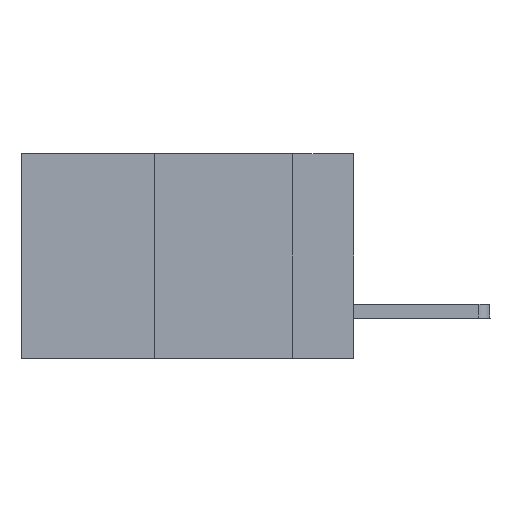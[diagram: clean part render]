
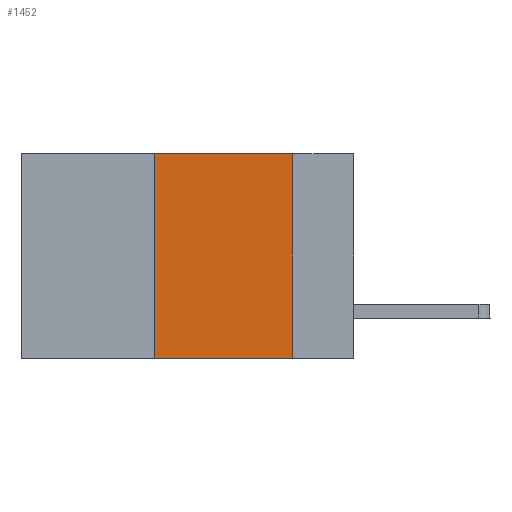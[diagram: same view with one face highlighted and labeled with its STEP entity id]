
A CAD part, left-side view. The second image highlights one B-rep face of the part: STEP entity #1452.
In plain terms, the highlighted planar face has unit normal (-1, 0, 0).
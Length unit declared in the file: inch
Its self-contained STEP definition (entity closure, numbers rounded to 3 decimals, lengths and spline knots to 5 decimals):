
#301 = DIRECTION ( 'NONE',  ( 1., 0., 0. ) ) ;
#927 = VERTEX_POINT ( 'NONE', #1703 ) ;
#1042 = EDGE_CURVE ( 'NONE', #5580, #927, #5784, .T. ) ;
#1264 = LINE ( 'NONE', #8928, #13347 ) ;
#1402 = VERTEX_POINT ( 'NONE', #9039 ) ;
#1452 = ADVANCED_FACE ( 'NONE', ( #6966 ), #12421, .F. ) ;
#1644 = VECTOR ( 'NONE', #13231, 39.37008 ) ;
#1703 = CARTESIAN_POINT ( 'NONE',  ( 0., 0.11, -0.37 ) ) ;
#1788 = ORIENTED_EDGE ( 'NONE', *, *, #7655, .F. ) ;
#1810 = VERTEX_POINT ( 'NONE', #11685 ) ;
#2211 = CARTESIAN_POINT ( 'NONE',  ( 0., 0.36, -0.37 ) ) ;
#3725 = DIRECTION ( 'NONE',  ( 0., -1., 0. ) ) ;
#4322 = AXIS2_PLACEMENT_3D ( 'NONE', #13526, #301, #13569 ) ;
#4919 = ORIENTED_EDGE ( 'NONE', *, *, #9323, .F. ) ;
#5501 = CARTESIAN_POINT ( 'NONE',  ( 0., 0.11, 0. ) ) ;
#5580 = VERTEX_POINT ( 'NONE', #2211 ) ;
#5591 = VECTOR ( 'NONE', #12750, 39.37008 ) ;
#5784 = LINE ( 'NONE', #10345, #8171 ) ;
#5958 = LINE ( 'NONE', #7363, #5591 ) ;
#6367 = ORIENTED_EDGE ( 'NONE', *, *, #9769, .F. ) ;
#6966 = FACE_OUTER_BOUND ( 'NONE', #12284, .T. ) ;
#7363 = CARTESIAN_POINT ( 'NONE',  ( 0., 0.36, 0. ) ) ;
#7487 = LINE ( 'NONE', #5501, #1644 ) ;
#7655 = EDGE_CURVE ( 'NONE', #1810, #927, #7487, .T. ) ;
#8171 = VECTOR ( 'NONE', #3725, 39.37008 ) ;
#8928 = CARTESIAN_POINT ( 'NONE',  ( 0., 0.6, 0. ) ) ;
#9039 = CARTESIAN_POINT ( 'NONE',  ( 0., 0.36, 0. ) ) ;
#9323 = EDGE_CURVE ( 'NONE', #1402, #1810, #1264, .T. ) ;
#9769 = EDGE_CURVE ( 'NONE', #5580, #1402, #5958, .T. ) ;
#9910 = DIRECTION ( 'NONE',  ( 0., -1., 0. ) ) ;
#10345 = CARTESIAN_POINT ( 'NONE',  ( 0., 0.6, -0.37 ) ) ;
#11685 = CARTESIAN_POINT ( 'NONE',  ( 0., 0.11, 0. ) ) ;
#12284 = EDGE_LOOP ( 'NONE', ( #1788, #4919, #6367, #12964 ) ) ;
#12421 = PLANE ( 'NONE',  #4322 ) ;
#12750 = DIRECTION ( 'NONE',  ( 0., 0., 1. ) ) ;
#12964 = ORIENTED_EDGE ( 'NONE', *, *, #1042, .T. ) ;
#13231 = DIRECTION ( 'NONE',  ( 0., 0., -1. ) ) ;
#13347 = VECTOR ( 'NONE', #9910, 39.37008 ) ;
#13526 = CARTESIAN_POINT ( 'NONE',  ( 0., 0.6, 0. ) ) ;
#13569 = DIRECTION ( 'NONE',  ( 0., 0., -1. ) ) ;
